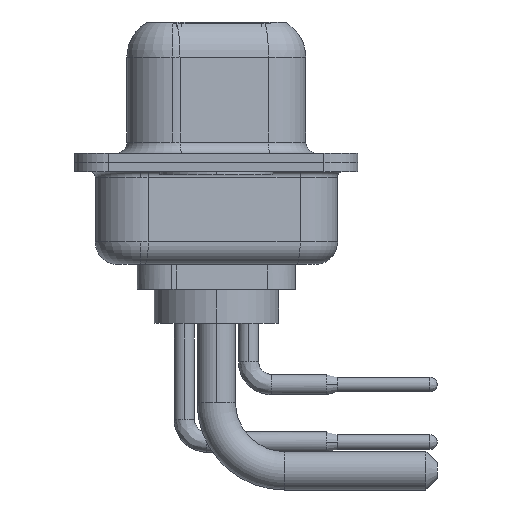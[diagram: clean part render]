
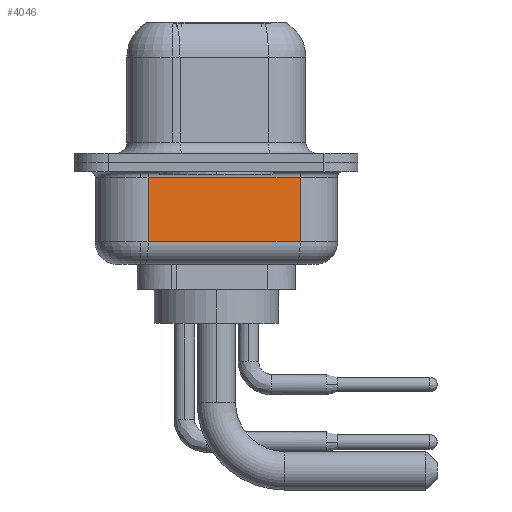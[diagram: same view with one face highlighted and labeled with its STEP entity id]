
A CAD part, left-side view. The second image highlights one B-rep face of the part: STEP entity #4046.
In plain terms, the highlighted planar face has unit normal (-0.985, -0.174, 0).
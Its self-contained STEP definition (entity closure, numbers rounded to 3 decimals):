
#52 = VECTOR ( 'NONE', #15308, 1000. ) ;
#83 = CARTESIAN_POINT ( 'NONE',  ( 2.855, 3.003, -4.5 ) ) ;
#539 = AXIS2_PLACEMENT_3D ( 'NONE', #83, #4800, #10532 ) ;
#829 = EDGE_CURVE ( 'NONE', #5471, #13359, #17366, .T. ) ;
#983 = CARTESIAN_POINT ( 'NONE',  ( 2.855, 3.003, -3.5 ) ) ;
#2404 = CARTESIAN_POINT ( 'NONE',  ( 2.855, 3.003, -0.65 ) ) ;
#2435 = DIRECTION ( 'NONE',  ( 0.174, -0.985, 0. ) ) ;
#2486 = CARTESIAN_POINT ( 'NONE',  ( 4.037, -3.697, -0.65 ) ) ;
#2670 = VECTOR ( 'NONE', #4006, 1000. ) ;
#2923 = VERTEX_POINT ( 'NONE', #2486 ) ;
#3356 = FACE_OUTER_BOUND ( 'NONE', #10192, .T. ) ;
#4006 = DIRECTION ( 'NONE',  ( 0., 0., 1. ) ) ;
#4046 = ADVANCED_FACE ( 'NONE', ( #3356 ), #4614, .F. ) ;
#4614 = PLANE ( 'NONE',  #539 ) ;
#4800 = DIRECTION ( 'NONE',  ( 0.985, 0.174, 0. ) ) ;
#5029 = ORIENTED_EDGE ( 'NONE', *, *, #15628, .T. ) ;
#5124 = ORIENTED_EDGE ( 'NONE', *, *, #9133, .F. ) ;
#5471 = VERTEX_POINT ( 'NONE', #10170 ) ;
#9082 = VECTOR ( 'NONE', #2435, 1000. ) ;
#9133 = EDGE_CURVE ( 'NONE', #5471, #18831, #9563, .T. ) ;
#9460 = CARTESIAN_POINT ( 'NONE',  ( 2.855, 3.003, -4.5 ) ) ;
#9563 = LINE ( 'NONE', #9460, #52 ) ;
#9749 = DIRECTION ( 'NONE',  ( -0.174, 0.985, 0. ) ) ;
#10009 = CARTESIAN_POINT ( 'NONE',  ( 4.037, -3.697, -4.5 ) ) ;
#10170 = CARTESIAN_POINT ( 'NONE',  ( 2.855, 3.003, -3.5 ) ) ;
#10192 = EDGE_LOOP ( 'NONE', ( #5124, #17672, #5029, #13714 ) ) ;
#10494 = CARTESIAN_POINT ( 'NONE',  ( 2.855, 3.003, -0.65 ) ) ;
#10532 = DIRECTION ( 'NONE',  ( -0.174, 0.985, 0. ) ) ;
#11455 = LINE ( 'NONE', #10009, #2670 ) ;
#13359 = VERTEX_POINT ( 'NONE', #15018 ) ;
#13581 = EDGE_CURVE ( 'NONE', #2923, #18831, #18777, .T. ) ;
#13714 = ORIENTED_EDGE ( 'NONE', *, *, #13581, .T. ) ;
#15018 = CARTESIAN_POINT ( 'NONE',  ( 4.037, -3.697, -3.5 ) ) ;
#15308 = DIRECTION ( 'NONE',  ( 0., 0., 1. ) ) ;
#15628 = EDGE_CURVE ( 'NONE', #13359, #2923, #11455, .T. ) ;
#16493 = VECTOR ( 'NONE', #9749, 1000. ) ;
#17366 = LINE ( 'NONE', #983, #9082 ) ;
#17672 = ORIENTED_EDGE ( 'NONE', *, *, #829, .T. ) ;
#18777 = LINE ( 'NONE', #2404, #16493 ) ;
#18831 = VERTEX_POINT ( 'NONE', #10494 ) ;
